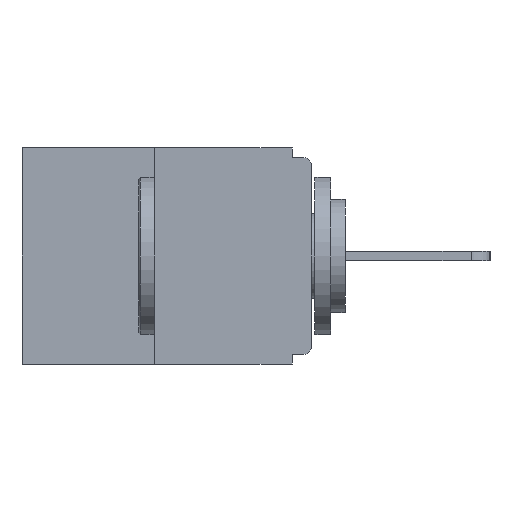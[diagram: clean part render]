
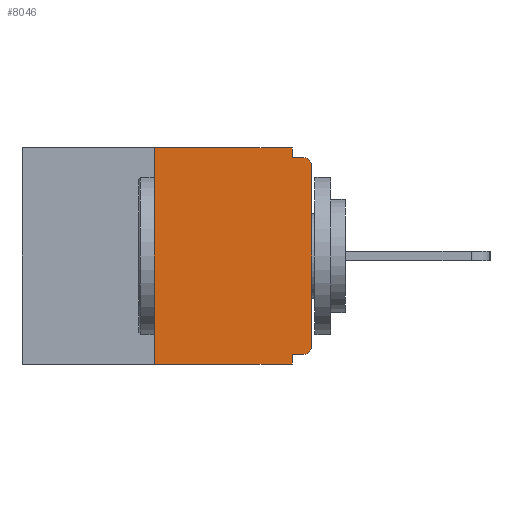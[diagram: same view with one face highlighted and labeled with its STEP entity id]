
A CAD part, left-side view. The second image highlights one B-rep face of the part: STEP entity #8046.
In plain terms, the highlighted planar face has unit normal (-1, 0, 0).
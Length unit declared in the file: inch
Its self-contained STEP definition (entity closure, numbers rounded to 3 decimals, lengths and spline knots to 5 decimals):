
#144 = VERTEX_POINT ( 'NONE', #12881 ) ;
#165 = CARTESIAN_POINT ( 'NONE',  ( 0., 0.46, -0.343 ) ) ;
#767 = EDGE_CURVE ( 'NONE', #5290, #12160, #3453, .T. ) ;
#1072 = DIRECTION ( 'NONE',  ( 0., -1., 0. ) ) ;
#1189 = ORIENTED_EDGE ( 'NONE', *, *, #767, .F. ) ;
#1317 = CARTESIAN_POINT ( 'NONE',  ( 0., 0.46, 0. ) ) ;
#1407 = FACE_OUTER_BOUND ( 'NONE', #8284, .T. ) ;
#1431 = CARTESIAN_POINT ( 'NONE',  ( 0., 0.031, -0.343 ) ) ;
#1513 = CIRCLE ( 'NONE', #2325, 0.015 ) ;
#1544 = DIRECTION ( 'NONE',  ( 0., -1., 0. ) ) ;
#1545 = EDGE_CURVE ( 'NONE', #5290, #10282, #5119, .T. ) ;
#1547 = ORIENTED_EDGE ( 'NONE', *, *, #2299, .F. ) ;
#1966 = VERTEX_POINT ( 'NONE', #6101 ) ;
#2023 = CARTESIAN_POINT ( 'NONE',  ( 0., 0.031, -0.015 ) ) ;
#2143 = VECTOR ( 'NONE', #11706, 39.37008 ) ;
#2187 = EDGE_CURVE ( 'NONE', #1966, #5656, #13552, .T. ) ;
#2299 = EDGE_CURVE ( 'NONE', #5656, #10282, #4575, .T. ) ;
#2325 = AXIS2_PLACEMENT_3D ( 'NONE', #5490, #12776, #6566 ) ;
#2876 = CARTESIAN_POINT ( 'NONE',  ( 0., 0.031, 0. ) ) ;
#3097 = EDGE_CURVE ( 'NONE', #144, #11832, #7244, .T. ) ;
#3274 = CARTESIAN_POINT ( 'NONE',  ( 0., 0.25, -0.343 ) ) ;
#3421 = EDGE_CURVE ( 'NONE', #11832, #13884, #13683, .T. ) ;
#3453 = LINE ( 'NONE', #5888, #9456 ) ;
#4207 = ORIENTED_EDGE ( 'NONE', *, *, #1545, .T. ) ;
#4352 = DIRECTION ( 'NONE',  ( 0., 0., -1. ) ) ;
#4529 = ORIENTED_EDGE ( 'NONE', *, *, #2187, .F. ) ;
#4575 = LINE ( 'NONE', #9713, #7099 ) ;
#4741 = CARTESIAN_POINT ( 'NONE',  ( 0., 0.25, 0. ) ) ;
#4865 = ORIENTED_EDGE ( 'NONE', *, *, #10072, .T. ) ;
#4896 = DIRECTION ( 'NONE',  ( 0., 0., 1. ) ) ;
#5119 = LINE ( 'NONE', #165, #2143 ) ;
#5221 = VECTOR ( 'NONE', #1072, 39.37008 ) ;
#5290 = VERTEX_POINT ( 'NONE', #3274 ) ;
#5490 = CARTESIAN_POINT ( 'NONE',  ( 0., 0.015, -0.03 ) ) ;
#5537 = CARTESIAN_POINT ( 'NONE',  ( 0., 0.031, -0.328 ) ) ;
#5656 = VERTEX_POINT ( 'NONE', #5537 ) ;
#5888 = CARTESIAN_POINT ( 'NONE',  ( 0., 0.25, 0. ) ) ;
#5892 = CARTESIAN_POINT ( 'NONE',  ( 0., 0., -0.015 ) ) ;
#6101 = CARTESIAN_POINT ( 'NONE',  ( 0., 0.015, -0.328 ) ) ;
#6231 = ORIENTED_EDGE ( 'NONE', *, *, #3097, .F. ) ;
#6566 = DIRECTION ( 'NONE',  ( 0., 0., -1. ) ) ;
#6596 = DIRECTION ( 'NONE',  ( -1., 0., 0. ) ) ;
#6723 = ORIENTED_EDGE ( 'NONE', *, *, #9061, .F. ) ;
#7099 = VECTOR ( 'NONE', #9679, 39.37008 ) ;
#7244 = LINE ( 'NONE', #2876, #12432 ) ;
#7853 = EDGE_CURVE ( 'NONE', #10635, #10499, #9243, .T. ) ;
#8046 = ADVANCED_FACE ( 'NONE', ( #1407 ), #8389, .F. ) ;
#8051 = LINE ( 'NONE', #1317, #5221 ) ;
#8284 = EDGE_LOOP ( 'NONE', ( #6723, #1189, #4207, #1547, #4529, #4865, #10507, #10826, #11463, #6231 ) ) ;
#8360 = DIRECTION ( 'NONE',  ( 0., 0., -1. ) ) ;
#8370 = DIRECTION ( 'NONE',  ( 1., 0., 0. ) ) ;
#8389 = PLANE ( 'NONE',  #9190 ) ;
#8492 = CARTESIAN_POINT ( 'NONE',  ( 0., 0.46, 0. ) ) ;
#8841 = CIRCLE ( 'NONE', #12891, 0.015 ) ;
#8907 = CARTESIAN_POINT ( 'NONE',  ( 0., 0.015, -0.015 ) ) ;
#9061 = EDGE_CURVE ( 'NONE', #12160, #144, #8051, .T. ) ;
#9190 = AXIS2_PLACEMENT_3D ( 'NONE', #8492, #8370, #8360 ) ;
#9243 = LINE ( 'NONE', #9954, #9571 ) ;
#9456 = VECTOR ( 'NONE', #4896, 39.37008 ) ;
#9571 = VECTOR ( 'NONE', #9935, 39.37008 ) ;
#9679 = DIRECTION ( 'NONE',  ( 0., 0., -1. ) ) ;
#9713 = CARTESIAN_POINT ( 'NONE',  ( 0., 0.031, -0.343 ) ) ;
#9935 = DIRECTION ( 'NONE',  ( 0., 0., 1. ) ) ;
#9954 = CARTESIAN_POINT ( 'NONE',  ( 0., 0., 0. ) ) ;
#10072 = EDGE_CURVE ( 'NONE', #1966, #10635, #8841, .T. ) ;
#10282 = VERTEX_POINT ( 'NONE', #1431 ) ;
#10461 = CARTESIAN_POINT ( 'NONE',  ( 0., 0., -0.03 ) ) ;
#10499 = VERTEX_POINT ( 'NONE', #10461 ) ;
#10507 = ORIENTED_EDGE ( 'NONE', *, *, #7853, .T. ) ;
#10635 = VERTEX_POINT ( 'NONE', #10671 ) ;
#10671 = CARTESIAN_POINT ( 'NONE',  ( 0., 0., -0.313 ) ) ;
#10826 = ORIENTED_EDGE ( 'NONE', *, *, #11270, .T. ) ;
#10871 = VECTOR ( 'NONE', #11561, 39.37008 ) ;
#11270 = EDGE_CURVE ( 'NONE', #10499, #13884, #1513, .T. ) ;
#11463 = ORIENTED_EDGE ( 'NONE', *, *, #3421, .F. ) ;
#11561 = DIRECTION ( 'NONE',  ( 0., 1., 0. ) ) ;
#11706 = DIRECTION ( 'NONE',  ( 0., -1., 0. ) ) ;
#11832 = VERTEX_POINT ( 'NONE', #2023 ) ;
#12160 = VERTEX_POINT ( 'NONE', #4741 ) ;
#12217 = CARTESIAN_POINT ( 'NONE',  ( 0., 0., -0.328 ) ) ;
#12432 = VECTOR ( 'NONE', #4352, 39.37008 ) ;
#12776 = DIRECTION ( 'NONE',  ( -1., 0., 0. ) ) ;
#12812 = CARTESIAN_POINT ( 'NONE',  ( 0., 0.015, -0.313 ) ) ;
#12881 = CARTESIAN_POINT ( 'NONE',  ( 0., 0.031, 0. ) ) ;
#12891 = AXIS2_PLACEMENT_3D ( 'NONE', #12812, #6596, #13813 ) ;
#13047 = VECTOR ( 'NONE', #1544, 39.37008 ) ;
#13552 = LINE ( 'NONE', #12217, #10871 ) ;
#13683 = LINE ( 'NONE', #5892, #13047 ) ;
#13813 = DIRECTION ( 'NONE',  ( 0., 0., -1. ) ) ;
#13884 = VERTEX_POINT ( 'NONE', #8907 ) ;
